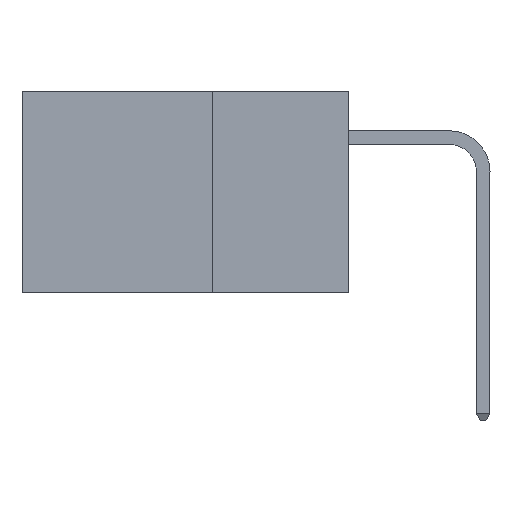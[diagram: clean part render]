
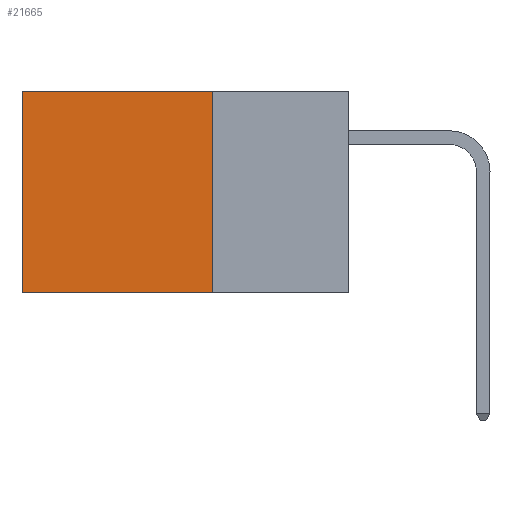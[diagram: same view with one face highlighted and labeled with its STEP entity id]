
A CAD part, left-side view. The second image highlights one B-rep face of the part: STEP entity #21665.
In plain terms, the highlighted planar face has unit normal (-1, 0, 0).
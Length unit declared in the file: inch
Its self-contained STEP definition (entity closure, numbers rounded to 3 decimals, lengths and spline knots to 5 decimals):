
#14 = CARTESIAN_POINT ( 'NONE',  ( 0.2875, 0.6, -0.37 ) ) ;
#484 = ORIENTED_EDGE ( 'NONE', *, *, #4555, .T. ) ;
#485 = CARTESIAN_POINT ( 'NONE',  ( 0.2875, 0.6, 0. ) ) ;
#1348 = LINE ( 'NONE', #26043, #14504 ) ;
#3463 = VERTEX_POINT ( 'NONE', #3578 ) ;
#3578 = CARTESIAN_POINT ( 'NONE',  ( 0.2875, 0.25, 0. ) ) ;
#3967 = DIRECTION ( 'NONE',  ( 0., 0., -1. ) ) ;
#4268 = PLANE ( 'NONE',  #31456 ) ;
#4554 = CARTESIAN_POINT ( 'NONE',  ( 0.2875, 0.25, -0.37 ) ) ;
#4555 = EDGE_CURVE ( 'NONE', #12743, #9274, #30809, .T. ) ;
#4929 = LINE ( 'NONE', #26466, #11947 ) ;
#5085 = ORIENTED_EDGE ( 'NONE', *, *, #35826, .T. ) ;
#9274 = VERTEX_POINT ( 'NONE', #14 ) ;
#11015 = DIRECTION ( 'NONE',  ( 0., 1., 0. ) ) ;
#11386 = FACE_OUTER_BOUND ( 'NONE', #34291, .T. ) ;
#11651 = DIRECTION ( 'NONE',  ( 0., 1., 0. ) ) ;
#11947 = VECTOR ( 'NONE', #38624, 39.37008 ) ;
#12743 = VERTEX_POINT ( 'NONE', #485 ) ;
#12869 = CARTESIAN_POINT ( 'NONE',  ( 0.2875, 0.6, 0. ) ) ;
#13306 = DIRECTION ( 'NONE',  ( 1., 0., 0. ) ) ;
#14504 = VECTOR ( 'NONE', #11015, 39.37008 ) ;
#17454 = CARTESIAN_POINT ( 'NONE',  ( 0.2875, 0.25, -0.37 ) ) ;
#20646 = ORIENTED_EDGE ( 'NONE', *, *, #32357, .F. ) ;
#21665 = ADVANCED_FACE ( 'NONE', ( #11386 ), #4268, .F. ) ;
#22810 = VECTOR ( 'NONE', #3967, 39.37008 ) ;
#26043 = CARTESIAN_POINT ( 'NONE',  ( 0.2875, 0.25, 0. ) ) ;
#26466 = CARTESIAN_POINT ( 'NONE',  ( 0.2875, 0.25, 0. ) ) ;
#27775 = VECTOR ( 'NONE', #11651, 39.37008 ) ;
#28717 = LINE ( 'NONE', #17454, #27775 ) ;
#29172 = EDGE_CURVE ( 'NONE', #34559, #9274, #28717, .T. ) ;
#30809 = LINE ( 'NONE', #12869, #22810 ) ;
#31154 = ORIENTED_EDGE ( 'NONE', *, *, #29172, .F. ) ;
#31361 = CARTESIAN_POINT ( 'NONE',  ( 0.2875, 0.25, 0. ) ) ;
#31456 = AXIS2_PLACEMENT_3D ( 'NONE', #31361, #13306, #34348 ) ;
#32357 = EDGE_CURVE ( 'NONE', #3463, #34559, #4929, .T. ) ;
#34291 = EDGE_LOOP ( 'NONE', ( #484, #31154, #20646, #5085 ) ) ;
#34348 = DIRECTION ( 'NONE',  ( 0., 0., -1. ) ) ;
#34559 = VERTEX_POINT ( 'NONE', #4554 ) ;
#35826 = EDGE_CURVE ( 'NONE', #3463, #12743, #1348, .T. ) ;
#38624 = DIRECTION ( 'NONE',  ( 0., 0., -1. ) ) ;
